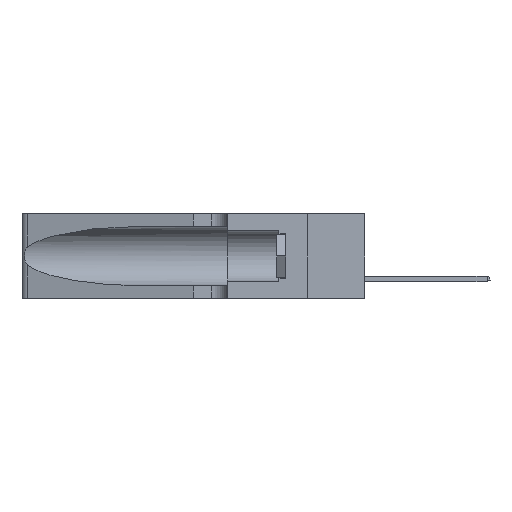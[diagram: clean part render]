
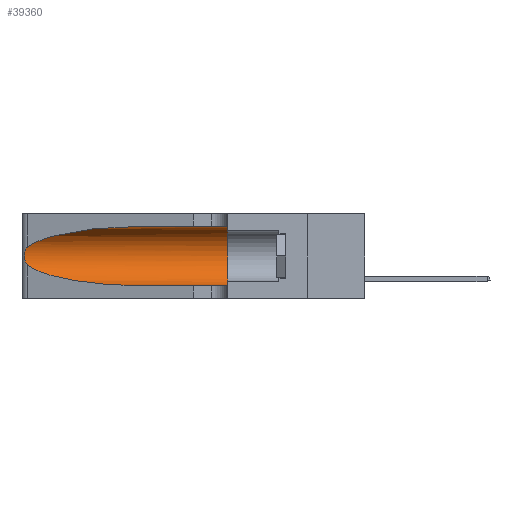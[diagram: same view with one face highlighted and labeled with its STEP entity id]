
A CAD part, left-side view. The second image highlights one B-rep face of the part: STEP entity #39360.
In plain terms, the highlighted cylindrical face has radius 3.308 mm (diameter 6.617 mm), a partial arc.
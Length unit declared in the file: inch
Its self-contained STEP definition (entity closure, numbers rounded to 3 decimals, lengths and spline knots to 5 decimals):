
#4304 = VERTEX_POINT ( 'NONE', #43884 ) ;
#5130 = CARTESIAN_POINT ( 'NONE',  ( 0.26018, 1.23835, 0.19895 ) ) ;
#5931 = CARTESIAN_POINT ( 'NONE',  ( 0.25487, 1.22718, 0.14631 ) ) ;
#6405 = ORIENTED_EDGE ( 'NONE', *, *, #44167, .T. ) ;
#7130 = DIRECTION ( 'NONE',  ( 0., -1., 0. ) ) ;
#7786 = LINE ( 'NONE', #30600, #47733 ) ;
#8189 = VERTEX_POINT ( 'NONE', #5931 ) ;
#9120 = CARTESIAN_POINT ( 'NONE',  ( 0.26075, 1.23896, 0.19203 ) ) ;
#10545 = CARTESIAN_POINT ( 'NONE',  ( 0.25639, 1.23186, 0.15144 ) ) ;
#10927 = VERTEX_POINT ( 'NONE', #34454 ) ;
#11132 = DIRECTION ( 'NONE',  ( 0., 1., 0. ) ) ;
#11928 =( BOUNDED_CURVE ( )  B_SPLINE_CURVE ( 3, ( #35945, #32254, #20139, #28356 ),
 .UNSPECIFIED., .F., .F. ) 
 B_SPLINE_CURVE_WITH_KNOTS ( ( 4, 4 ),
 ( 3.44316, 4.71239 ),
 .UNSPECIFIED. ) 
 CURVE ( )  GEOMETRIC_REPRESENTATION_ITEM ( )  RATIONAL_B_SPLINE_CURVE ( ( 1., 0.87, 0.87, 1. ) ) 
 REPRESENTATION_ITEM ( '' )  );
#12067 = CARTESIAN_POINT ( 'NONE',  ( 0.25487, 1.22718, 0.22369 ) ) ;
#12644 = EDGE_LOOP ( 'NONE', ( #21413, #49463, #6405, #45100, #21302, #17727 ) ) ;
#13304 = CARTESIAN_POINT ( 'NONE',  ( 0.26075, 1.23896, 0.178 ) ) ;
#15075 = DIRECTION ( 'NONE',  ( 0., -1., 0. ) ) ;
#15131 = DIRECTION ( 'NONE',  ( 0., 0., 1. ) ) ;
#17221 = B_SPLINE_CURVE_WITH_KNOTS ( 'NONE', 3,
 ( #12067, #39840, #23806, #20683, #40467, #5130, #9120, #13304, #50620, #20314, #20946, #10545, #47745, #40215 ),
 .UNSPECIFIED., .F., .F.,
 ( 4, 2, 2, 2, 2, 2, 4 ),
 ( 0., 0.00027, 0.00053, 0.00107, 0.0016, 0.00187, 0.00214 ),
 .UNSPECIFIED. ) ;
#17727 = ORIENTED_EDGE ( 'NONE', *, *, #20080, .F. ) ;
#18849 = DIRECTION ( 'NONE',  ( 0., -1., 0. ) ) ;
#20080 = EDGE_CURVE ( 'NONE', #4304, #49728, #30573, .T. ) ;
#20139 = CARTESIAN_POINT ( 'NONE',  ( 0.18966, 0.96281, 0.05475 ) ) ;
#20314 = CARTESIAN_POINT ( 'NONE',  ( 0.25856, 1.23593, 0.16098 ) ) ;
#20683 = CARTESIAN_POINT ( 'NONE',  ( 0.25787, 1.23484, 0.2124 ) ) ;
#20946 = CARTESIAN_POINT ( 'NONE',  ( 0.25789, 1.23486, 0.15765 ) ) ;
#21302 = ORIENTED_EDGE ( 'NONE', *, *, #28169, .F. ) ;
#21413 = ORIENTED_EDGE ( 'NONE', *, *, #26956, .T. ) ;
#23217 = CARTESIAN_POINT ( 'NONE',  ( 0.25487, 1.22718, 0.22369 ) ) ;
#23368 = VERTEX_POINT ( 'NONE', #30726 ) ;
#23806 = CARTESIAN_POINT ( 'NONE',  ( 0.25639, 1.23184, 0.21858 ) ) ;
#24261 = VECTOR ( 'NONE', #15075, 39.37008 ) ;
#25042 = CARTESIAN_POINT ( 'NONE',  ( 0.1305, 1.61858, 0.31525 ) ) ;
#26783 = CYLINDRICAL_SURFACE ( 'NONE', #27696, 0.13025 ) ;
#26956 = EDGE_CURVE ( 'NONE', #4304, #40734, #29454, .T. ) ;
#27405 = AXIS2_PLACEMENT_3D ( 'NONE', #31081, #11132, #15131 ) ;
#27667 = CARTESIAN_POINT ( 'NONE',  ( 0.1305, 0.35, 0.31525 ) ) ;
#27696 = AXIS2_PLACEMENT_3D ( 'NONE', #41224, #7130, #37811 ) ;
#28169 = EDGE_CURVE ( 'NONE', #49728, #10927, #41096, .T. ) ;
#28356 = CARTESIAN_POINT ( 'NONE',  ( 0.1305, 0.72297, 0.05475 ) ) ;
#29454 =( BOUNDED_CURVE ( )  B_SPLINE_CURVE ( 3, ( #32520, #42021, #50048, #23217 ),
 .UNSPECIFIED., .F., .F. ) 
 B_SPLINE_CURVE_WITH_KNOTS ( ( 4, 4 ),
 ( 1.5708, 2.84003 ),
 .UNSPECIFIED. ) 
 CURVE ( )  GEOMETRIC_REPRESENTATION_ITEM ( )  RATIONAL_B_SPLINE_CURVE ( ( 1., 0.87, 0.87, 1. ) ) 
 REPRESENTATION_ITEM ( '' )  );
#30573 = LINE ( 'NONE', #25042, #24261 ) ;
#30600 = CARTESIAN_POINT ( 'NONE',  ( 0.1305, 1.61858, 0.05475 ) ) ;
#30726 = CARTESIAN_POINT ( 'NONE',  ( 0.1305, 0.72297, 0.05475 ) ) ;
#31081 = CARTESIAN_POINT ( 'NONE',  ( 0.1305, 0.35, 0.185 ) ) ;
#32254 = CARTESIAN_POINT ( 'NONE',  ( 0.2373, 1.15595, 0.08982 ) ) ;
#32520 = CARTESIAN_POINT ( 'NONE',  ( 0.1305, 0.72297, 0.31525 ) ) ;
#34275 = CARTESIAN_POINT ( 'NONE',  ( 0.25487, 1.22718, 0.22369 ) ) ;
#34454 = CARTESIAN_POINT ( 'NONE',  ( 0.1305, 0.35, 0.05475 ) ) ;
#35945 = CARTESIAN_POINT ( 'NONE',  ( 0.25487, 1.22718, 0.14631 ) ) ;
#36363 = EDGE_CURVE ( 'NONE', #40734, #8189, #17221, .T. ) ;
#37811 = DIRECTION ( 'NONE',  ( 0., 0., -1. ) ) ;
#39360 = ADVANCED_FACE ( 'NONE', ( #41088 ), #26783, .F. ) ;
#39840 = CARTESIAN_POINT ( 'NONE',  ( 0.25555, 1.22994, 0.2215 ) ) ;
#40215 = CARTESIAN_POINT ( 'NONE',  ( 0.25487, 1.22718, 0.14631 ) ) ;
#40467 = CARTESIAN_POINT ( 'NONE',  ( 0.25854, 1.2359, 0.20912 ) ) ;
#40734 = VERTEX_POINT ( 'NONE', #34275 ) ;
#41088 = FACE_OUTER_BOUND ( 'NONE', #12644, .T. ) ;
#41096 = CIRCLE ( 'NONE', #27405, 0.13025 ) ;
#41224 = CARTESIAN_POINT ( 'NONE',  ( 0.1305, 1.61858, 0.185 ) ) ;
#41622 = EDGE_CURVE ( 'NONE', #23368, #10927, #7786, .T. ) ;
#42021 = CARTESIAN_POINT ( 'NONE',  ( 0.18966, 0.96281, 0.31525 ) ) ;
#43884 = CARTESIAN_POINT ( 'NONE',  ( 0.1305, 0.72297, 0.31525 ) ) ;
#44167 = EDGE_CURVE ( 'NONE', #8189, #23368, #11928, .T. ) ;
#45100 = ORIENTED_EDGE ( 'NONE', *, *, #41622, .T. ) ;
#47733 = VECTOR ( 'NONE', #18849, 39.37008 ) ;
#47745 = CARTESIAN_POINT ( 'NONE',  ( 0.25555, 1.22993, 0.14849 ) ) ;
#49463 = ORIENTED_EDGE ( 'NONE', *, *, #36363, .T. ) ;
#49728 = VERTEX_POINT ( 'NONE', #27667 ) ;
#50048 = CARTESIAN_POINT ( 'NONE',  ( 0.2373, 1.15595, 0.28018 ) ) ;
#50620 = CARTESIAN_POINT ( 'NONE',  ( 0.26017, 1.23833, 0.17102 ) ) ;
